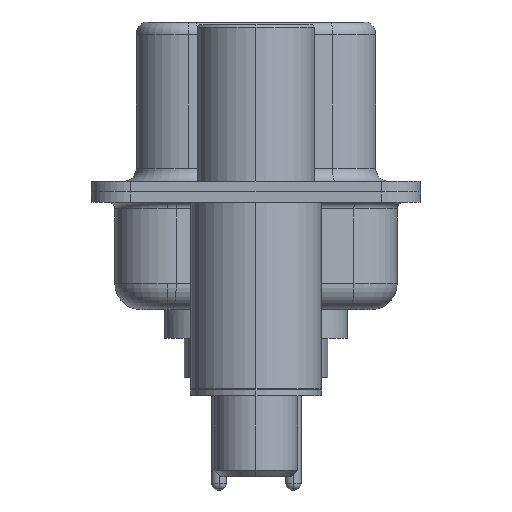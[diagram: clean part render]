
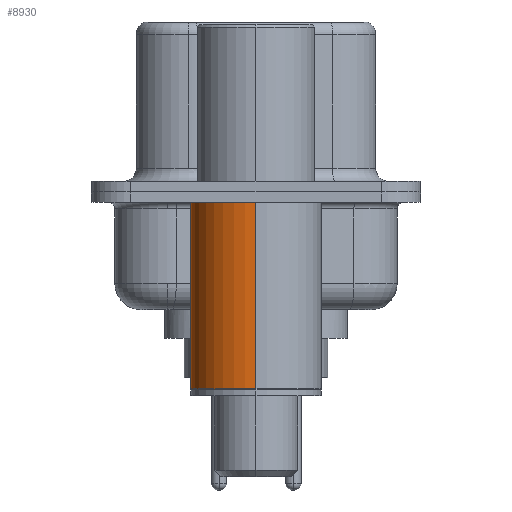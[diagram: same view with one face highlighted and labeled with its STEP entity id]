
A CAD part, left-side view. The second image highlights one B-rep face of the part: STEP entity #8930.
In plain terms, the highlighted cylindrical face has radius 2.5 mm (diameter 5 mm), a partial arc.
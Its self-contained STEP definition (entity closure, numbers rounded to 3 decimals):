
#536 = CIRCLE ( 'NONE', #8363, 2.5 ) ;
#700 = ORIENTED_EDGE ( 'NONE', *, *, #13765, .T. ) ;
#805 = ORIENTED_EDGE ( 'NONE', *, *, #13766, .F. ) ;
#2467 = DIRECTION ( 'NONE',  ( 1., 0., 0. ) ) ;
#2685 = VERTEX_POINT ( 'NONE', #11748 ) ;
#2698 = DIRECTION ( 'NONE',  ( 0., 0., 1. ) ) ;
#3809 = CARTESIAN_POINT ( 'NONE',  ( 2.5, 0., -0.4 ) ) ;
#3831 = LINE ( 'NONE', #17395, #14198 ) ;
#5411 = DIRECTION ( 'NONE',  ( 0., 0., 1. ) ) ;
#5538 = DIRECTION ( 'NONE',  ( 0., 0., 1. ) ) ;
#5796 = AXIS2_PLACEMENT_3D ( 'NONE', #10668, #7962, #2467 ) ;
#6808 = DIRECTION ( 'NONE',  ( 0., 0., 1. ) ) ;
#7289 = CARTESIAN_POINT ( 'NONE',  ( 2.5, 0., -7.525 ) ) ;
#7487 = CIRCLE ( 'NONE', #9251, 2.5 ) ;
#7962 = DIRECTION ( 'NONE',  ( 0., 0., 1. ) ) ;
#8363 = AXIS2_PLACEMENT_3D ( 'NONE', #13507, #5411, #14831 ) ;
#8712 = CYLINDRICAL_SURFACE ( 'NONE', #5796, 2.5 ) ;
#8930 = ADVANCED_FACE ( 'NONE', ( #15773 ), #8712, .T. ) ;
#9240 = CARTESIAN_POINT ( 'NONE',  ( -2.5, 0., -0.4 ) ) ;
#9251 = AXIS2_PLACEMENT_3D ( 'NONE', #10872, #2698, #12233 ) ;
#9807 = VECTOR ( 'NONE', #5538, 1000. ) ;
#10668 = CARTESIAN_POINT ( 'NONE',  ( 0., 0., 0.581 ) ) ;
#10711 = ORIENTED_EDGE ( 'NONE', *, *, #13741, .T. ) ;
#10872 = CARTESIAN_POINT ( 'NONE',  ( 0., 0., -0.4 ) ) ;
#11748 = CARTESIAN_POINT ( 'NONE',  ( -2.5, 0., -7.525 ) ) ;
#12233 = DIRECTION ( 'NONE',  ( 1., 0., 0. ) ) ;
#13023 = ORIENTED_EDGE ( 'NONE', *, *, #13788, .F. ) ;
#13263 = VERTEX_POINT ( 'NONE', #7289 ) ;
#13349 = LINE ( 'NONE', #13620, #9807 ) ;
#13507 = CARTESIAN_POINT ( 'NONE',  ( 0., 0., -7.525 ) ) ;
#13620 = CARTESIAN_POINT ( 'NONE',  ( 2.5, 0., 0.581 ) ) ;
#13672 = VERTEX_POINT ( 'NONE', #3809 ) ;
#13741 = EDGE_CURVE ( 'NONE', #13263, #2685, #536, .T. ) ;
#13765 = EDGE_CURVE ( 'NONE', #2685, #14575, #3831, .T. ) ;
#13766 = EDGE_CURVE ( 'NONE', #13672, #14575, #7487, .T. ) ;
#13788 = EDGE_CURVE ( 'NONE', #13263, #13672, #13349, .T. ) ;
#14198 = VECTOR ( 'NONE', #6808, 1000. ) ;
#14575 = VERTEX_POINT ( 'NONE', #9240 ) ;
#14831 = DIRECTION ( 'NONE',  ( 1., 0., 0. ) ) ;
#15773 = FACE_OUTER_BOUND ( 'NONE', #17195, .T. ) ;
#17195 = EDGE_LOOP ( 'NONE', ( #10711, #700, #805, #13023 ) ) ;
#17395 = CARTESIAN_POINT ( 'NONE',  ( -2.5, 0., 0.581 ) ) ;
